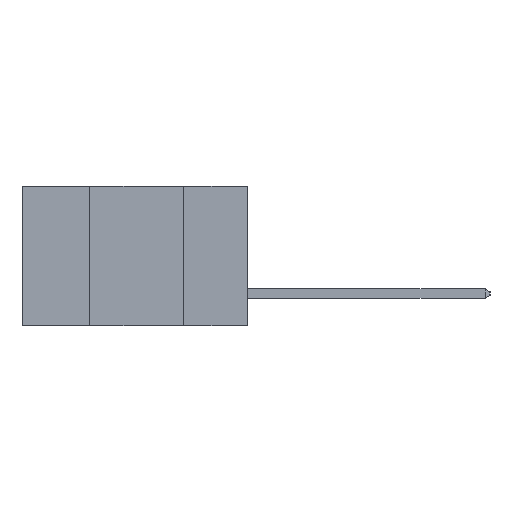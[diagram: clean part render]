
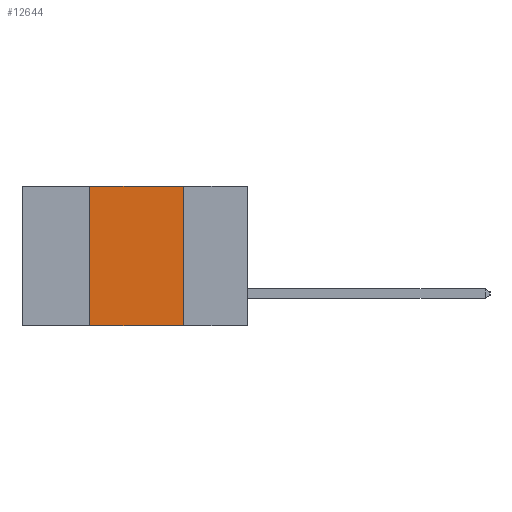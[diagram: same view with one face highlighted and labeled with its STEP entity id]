
A CAD part, left-side view. The second image highlights one B-rep face of the part: STEP entity #12644.
In plain terms, the highlighted planar face has unit normal (-1, 0, 0).
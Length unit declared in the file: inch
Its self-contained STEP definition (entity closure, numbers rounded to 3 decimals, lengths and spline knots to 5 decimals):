
#1 = AXIS2_PLACEMENT_3D ( 'NONE', #18831, #8926, #20453 ) ;
#336 = CARTESIAN_POINT ( 'NONE',  ( 0., 0.17, 0. ) ) ;
#414 = DIRECTION ( 'NONE',  ( 0., 0., -1. ) ) ;
#638 = VECTOR ( 'NONE', #414, 39.37008 ) ;
#653 = ORIENTED_EDGE ( 'NONE', *, *, #5468, .F. ) ;
#1805 = CARTESIAN_POINT ( 'NONE',  ( 0., 0.42, 0. ) ) ;
#2434 = CARTESIAN_POINT ( 'NONE',  ( 0., 0.17, 0. ) ) ;
#2514 = VECTOR ( 'NONE', #11598, 39.37008 ) ;
#2859 = CARTESIAN_POINT ( 'NONE',  ( 0., 0.17, -0.37 ) ) ;
#3433 = ORIENTED_EDGE ( 'NONE', *, *, #5271, .T. ) ;
#3920 = VECTOR ( 'NONE', #7571, 39.37008 ) ;
#4587 = LINE ( 'NONE', #12169, #8520 ) ;
#5271 = EDGE_CURVE ( 'NONE', #17716, #20506, #11891, .T. ) ;
#5440 = EDGE_CURVE ( 'NONE', #14212, #20506, #13926, .T. ) ;
#5468 = EDGE_CURVE ( 'NONE', #9217, #14212, #4587, .T. ) ;
#7571 = DIRECTION ( 'NONE',  ( 0., 0., 1. ) ) ;
#8520 = VECTOR ( 'NONE', #20364, 39.37008 ) ;
#8926 = DIRECTION ( 'NONE',  ( 1., 0., 0. ) ) ;
#9217 = VERTEX_POINT ( 'NONE', #1805 ) ;
#9975 = CARTESIAN_POINT ( 'NONE',  ( 0., 0.42, -0.37 ) ) ;
#10550 = FACE_OUTER_BOUND ( 'NONE', #16274, .T. ) ;
#11598 = DIRECTION ( 'NONE',  ( 0., -1., 0. ) ) ;
#11891 = LINE ( 'NONE', #18165, #2514 ) ;
#12169 = CARTESIAN_POINT ( 'NONE',  ( 0., 0.6, 0. ) ) ;
#12644 = ADVANCED_FACE ( 'NONE', ( #10550 ), #20380, .F. ) ;
#13441 = EDGE_CURVE ( 'NONE', #17716, #9217, #17152, .T. ) ;
#13926 = LINE ( 'NONE', #336, #638 ) ;
#14212 = VERTEX_POINT ( 'NONE', #2434 ) ;
#16274 = EDGE_LOOP ( 'NONE', ( #17486, #653, #17456, #3433 ) ) ;
#17152 = LINE ( 'NONE', #19140, #3920 ) ;
#17456 = ORIENTED_EDGE ( 'NONE', *, *, #13441, .F. ) ;
#17486 = ORIENTED_EDGE ( 'NONE', *, *, #5440, .F. ) ;
#17716 = VERTEX_POINT ( 'NONE', #9975 ) ;
#18165 = CARTESIAN_POINT ( 'NONE',  ( 0., 0.6, -0.37 ) ) ;
#18831 = CARTESIAN_POINT ( 'NONE',  ( 0., 0.6, 0. ) ) ;
#19140 = CARTESIAN_POINT ( 'NONE',  ( 0., 0.42, 0. ) ) ;
#20364 = DIRECTION ( 'NONE',  ( 0., -1., 0. ) ) ;
#20380 = PLANE ( 'NONE',  #1 ) ;
#20453 = DIRECTION ( 'NONE',  ( 0., 0., -1. ) ) ;
#20506 = VERTEX_POINT ( 'NONE', #2859 ) ;
